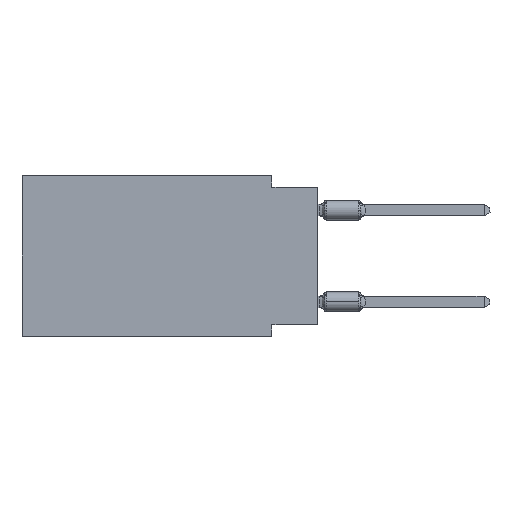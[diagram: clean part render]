
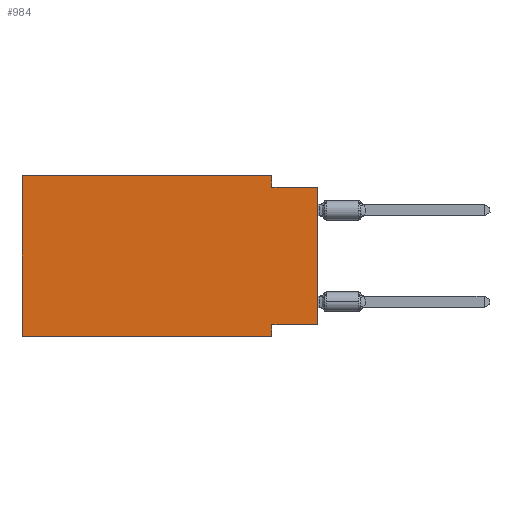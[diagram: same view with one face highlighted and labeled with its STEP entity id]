
A CAD part, left-side view. The second image highlights one B-rep face of the part: STEP entity #984.
In plain terms, the highlighted planar face has unit normal (-1, 0, 0).
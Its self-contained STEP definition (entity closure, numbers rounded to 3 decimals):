
#321 = EDGE_CURVE ( 'NONE', #17028, #18931, #11105, .T. ) ;
#624 = VECTOR ( 'NONE', #10607, 1000. ) ;
#938 = CARTESIAN_POINT ( 'NONE',  ( 0., 0., -0.635 ) ) ;
#984 = ADVANCED_FACE ( 'NONE', ( #22178 ), #26721, .F. ) ;
#1116 = CARTESIAN_POINT ( 'NONE',  ( 0., 0., -0.635 ) ) ;
#1461 = VERTEX_POINT ( 'NONE', #6932 ) ;
#2117 = VERTEX_POINT ( 'NONE', #28542 ) ;
#2151 = DIRECTION ( 'NONE',  ( 0., 0., -1. ) ) ;
#3022 = VERTEX_POINT ( 'NONE', #11292 ) ;
#3024 = CARTESIAN_POINT ( 'NONE',  ( 0., 16.383, 0. ) ) ;
#5759 = DIRECTION ( 'NONE',  ( 0., -1., 0. ) ) ;
#5932 = VECTOR ( 'NONE', #7495, 1000. ) ;
#6139 = CARTESIAN_POINT ( 'NONE',  ( 0., 16.383, 0. ) ) ;
#6932 = CARTESIAN_POINT ( 'NONE',  ( 0., 2.54, -8.89 ) ) ;
#7120 = EDGE_LOOP ( 'NONE', ( #20575, #7157, #21048, #24520, #26034, #12114, #10329, #11367 ) ) ;
#7157 = ORIENTED_EDGE ( 'NONE', *, *, #15041, .F. ) ;
#7402 = DIRECTION ( 'NONE',  ( 0., 0., -1. ) ) ;
#7495 = DIRECTION ( 'NONE',  ( 0., 0., -1. ) ) ;
#7819 = VECTOR ( 'NONE', #16638, 1000. ) ;
#10251 = DIRECTION ( 'NONE',  ( 0., 0., 1. ) ) ;
#10329 = ORIENTED_EDGE ( 'NONE', *, *, #18226, .F. ) ;
#10607 = DIRECTION ( 'NONE',  ( 0., 0., 1. ) ) ;
#10887 = VERTEX_POINT ( 'NONE', #1116 ) ;
#11105 = LINE ( 'NONE', #17544, #19694 ) ;
#11111 = VECTOR ( 'NONE', #2151, 1000. ) ;
#11292 = CARTESIAN_POINT ( 'NONE',  ( 0., 2.54, 0. ) ) ;
#11367 = ORIENTED_EDGE ( 'NONE', *, *, #321, .F. ) ;
#11460 = EDGE_CURVE ( 'NONE', #17028, #10887, #17478, .T. ) ;
#11660 = VECTOR ( 'NONE', #10251, 1000. ) ;
#12114 = ORIENTED_EDGE ( 'NONE', *, *, #17282, .T. ) ;
#12349 = CARTESIAN_POINT ( 'NONE',  ( 0., 2.54, -8.255 ) ) ;
#13765 = CARTESIAN_POINT ( 'NONE',  ( 0., 0., 0. ) ) ;
#13945 = CARTESIAN_POINT ( 'NONE',  ( 0., 2.54, 0. ) ) ;
#14009 = LINE ( 'NONE', #22929, #7819 ) ;
#14191 = VERTEX_POINT ( 'NONE', #18586 ) ;
#15041 = EDGE_CURVE ( 'NONE', #2117, #10887, #18789, .T. ) ;
#15471 = EDGE_CURVE ( 'NONE', #27643, #14191, #21360, .T. ) ;
#15558 = AXIS2_PLACEMENT_3D ( 'NONE', #23046, #27451, #7402 ) ;
#16638 = DIRECTION ( 'NONE',  ( 0., -1., 0. ) ) ;
#17028 = VERTEX_POINT ( 'NONE', #22049 ) ;
#17282 = EDGE_CURVE ( 'NONE', #27643, #1461, #14009, .T. ) ;
#17478 = LINE ( 'NONE', #13765, #624 ) ;
#17544 = CARTESIAN_POINT ( 'NONE',  ( 0., 0., -8.255 ) ) ;
#17556 = EDGE_CURVE ( 'NONE', #3022, #2117, #20801, .T. ) ;
#17692 = DIRECTION ( 'NONE',  ( 0., 1., 0. ) ) ;
#18226 = EDGE_CURVE ( 'NONE', #18931, #1461, #22054, .T. ) ;
#18586 = CARTESIAN_POINT ( 'NONE',  ( 0., 16.383, 0. ) ) ;
#18789 = LINE ( 'NONE', #938, #22387 ) ;
#18931 = VERTEX_POINT ( 'NONE', #12349 ) ;
#19694 = VECTOR ( 'NONE', #17692, 1000. ) ;
#19708 = EDGE_CURVE ( 'NONE', #14191, #3022, #21019, .T. ) ;
#20575 = ORIENTED_EDGE ( 'NONE', *, *, #11460, .T. ) ;
#20801 = LINE ( 'NONE', #13945, #5932 ) ;
#21019 = LINE ( 'NONE', #3024, #28292 ) ;
#21048 = ORIENTED_EDGE ( 'NONE', *, *, #17556, .F. ) ;
#21360 = LINE ( 'NONE', #6139, #11660 ) ;
#22049 = CARTESIAN_POINT ( 'NONE',  ( 0., 0., -8.255 ) ) ;
#22054 = LINE ( 'NONE', #28811, #11111 ) ;
#22178 = FACE_OUTER_BOUND ( 'NONE', #7120, .T. ) ;
#22387 = VECTOR ( 'NONE', #5759, 1000. ) ;
#22929 = CARTESIAN_POINT ( 'NONE',  ( 0., 16.383, -8.89 ) ) ;
#23046 = CARTESIAN_POINT ( 'NONE',  ( 0., 16.383, 0. ) ) ;
#24520 = ORIENTED_EDGE ( 'NONE', *, *, #19708, .F. ) ;
#25375 = CARTESIAN_POINT ( 'NONE',  ( 0., 16.383, -8.89 ) ) ;
#25713 = DIRECTION ( 'NONE',  ( 0., -1., 0. ) ) ;
#26034 = ORIENTED_EDGE ( 'NONE', *, *, #15471, .F. ) ;
#26721 = PLANE ( 'NONE',  #15558 ) ;
#27451 = DIRECTION ( 'NONE',  ( 1., 0., 0. ) ) ;
#27643 = VERTEX_POINT ( 'NONE', #25375 ) ;
#28292 = VECTOR ( 'NONE', #25713, 1000. ) ;
#28542 = CARTESIAN_POINT ( 'NONE',  ( 0., 2.54, -0.635 ) ) ;
#28811 = CARTESIAN_POINT ( 'NONE',  ( 0., 2.54, -8.89 ) ) ;
